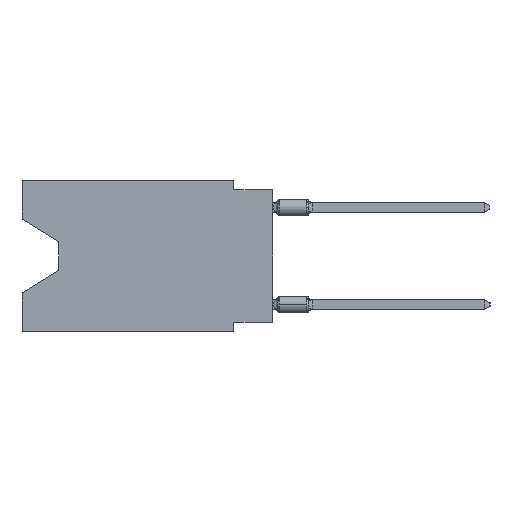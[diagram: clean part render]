
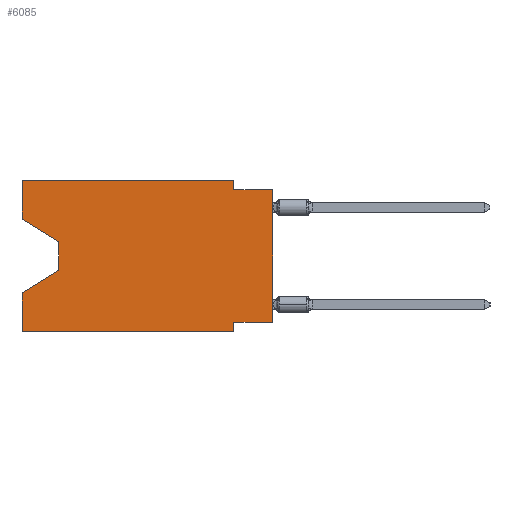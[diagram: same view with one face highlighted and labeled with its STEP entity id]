
A CAD part, left-side view. The second image highlights one B-rep face of the part: STEP entity #6085.
In plain terms, the highlighted planar face has unit normal (-1, 0, 0).
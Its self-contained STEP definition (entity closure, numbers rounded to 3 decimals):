
#552 = AXIS2_PLACEMENT_3D ( 'NONE', #18874, #6855, #30399 ) ;
#792 = EDGE_CURVE ( 'NONE', #24666, #30831, #25590, .T. ) ;
#1021 = CARTESIAN_POINT ( 'NONE',  ( 0., 16.383, -9.906 ) ) ;
#1111 = VERTEX_POINT ( 'NONE', #17667 ) ;
#1192 = VECTOR ( 'NONE', #21020, 1000. ) ;
#1238 = VECTOR ( 'NONE', #3742, 1000. ) ;
#1611 = ORIENTED_EDGE ( 'NONE', *, *, #27553, .F. ) ;
#3358 = DIRECTION ( 'NONE',  ( 0., 0., -1. ) ) ;
#3742 = DIRECTION ( 'NONE',  ( 0., -0.855, -0.519 ) ) ;
#4316 = EDGE_CURVE ( 'NONE', #13164, #8868, #20007, .T. ) ;
#6073 = DIRECTION ( 'NONE',  ( 0., 0., 1. ) ) ;
#6085 = ADVANCED_FACE ( 'NONE', ( #26122 ), #13973, .F. ) ;
#6560 = DIRECTION ( 'NONE',  ( 0., 0.855, -0.519 ) ) ;
#6799 = LINE ( 'NONE', #18811, #1192 ) ;
#6855 = DIRECTION ( 'NONE',  ( 1., 0., 0. ) ) ;
#7568 = VECTOR ( 'NONE', #22548, 1000. ) ;
#8240 = VERTEX_POINT ( 'NONE', #14431 ) ;
#8868 = VERTEX_POINT ( 'NONE', #10588 ) ;
#9000 = VECTOR ( 'NONE', #24006, 1000. ) ;
#9564 = EDGE_CURVE ( 'NONE', #27578, #13164, #17744, .T. ) ;
#9572 = ORIENTED_EDGE ( 'NONE', *, *, #4316, .F. ) ;
#10079 = CARTESIAN_POINT ( 'NONE',  ( 0., 16.383, -7.36 ) ) ;
#10084 = VECTOR ( 'NONE', #27283, 1000. ) ;
#10448 = ORIENTED_EDGE ( 'NONE', *, *, #28836, .T. ) ;
#10464 = DIRECTION ( 'NONE',  ( 0., 1., 0. ) ) ;
#10588 = CARTESIAN_POINT ( 'NONE',  ( 0., 2.54, -9.906 ) ) ;
#11157 = CARTESIAN_POINT ( 'NONE',  ( 0., 2.54, 0. ) ) ;
#11497 = EDGE_LOOP ( 'NONE', ( #19153, #28669, #14744, #1611, #18763, #9572, #24046, #10448, #26878, #20129, #12836, #22927 ) ) ;
#11610 = DIRECTION ( 'NONE',  ( 0., 0., 1. ) ) ;
#11919 = CARTESIAN_POINT ( 'NONE',  ( 0., 2.54, -0.635 ) ) ;
#12631 = CARTESIAN_POINT ( 'NONE',  ( 0., 16.383, 0. ) ) ;
#12836 = ORIENTED_EDGE ( 'NONE', *, *, #30346, .F. ) ;
#13164 = VERTEX_POINT ( 'NONE', #17005 ) ;
#13759 = DIRECTION ( 'NONE',  ( 0., 0., -1. ) ) ;
#13772 = VERTEX_POINT ( 'NONE', #1021 ) ;
#13973 = PLANE ( 'NONE',  #552 ) ;
#14310 = EDGE_CURVE ( 'NONE', #30289, #8240, #6799, .T. ) ;
#14431 = CARTESIAN_POINT ( 'NONE',  ( 0., 16.383, 0. ) ) ;
#14514 = LINE ( 'NONE', #24137, #17975 ) ;
#14744 = ORIENTED_EDGE ( 'NONE', *, *, #18075, .T. ) ;
#15206 = EDGE_CURVE ( 'NONE', #30289, #24666, #27894, .T. ) ;
#15303 = CARTESIAN_POINT ( 'NONE',  ( 0., 16.383, -9.906 ) ) ;
#15611 = LINE ( 'NONE', #15303, #7568 ) ;
#15722 = VECTOR ( 'NONE', #10464, 1000. ) ;
#15878 = CARTESIAN_POINT ( 'NONE',  ( 0., 0., 0. ) ) ;
#16184 = CARTESIAN_POINT ( 'NONE',  ( 0., 0., -9.271 ) ) ;
#16784 = VECTOR ( 'NONE', #13759, 1000. ) ;
#17005 = CARTESIAN_POINT ( 'NONE',  ( 0., 2.54, -9.271 ) ) ;
#17667 = CARTESIAN_POINT ( 'NONE',  ( 0., 0., -0.635 ) ) ;
#17744 = LINE ( 'NONE', #26477, #15722 ) ;
#17975 = VECTOR ( 'NONE', #21774, 1000. ) ;
#18075 = EDGE_CURVE ( 'NONE', #30831, #23262, #25360, .T. ) ;
#18541 = EDGE_CURVE ( 'NONE', #21445, #29987, #24992, .T. ) ;
#18633 = VECTOR ( 'NONE', #3358, 1000. ) ;
#18659 = CARTESIAN_POINT ( 'NONE',  ( 0., 13.97, -5.893 ) ) ;
#18763 = ORIENTED_EDGE ( 'NONE', *, *, #19671, .T. ) ;
#18811 = CARTESIAN_POINT ( 'NONE',  ( 0., 16.383, 0. ) ) ;
#18874 = CARTESIAN_POINT ( 'NONE',  ( 0., 16.383, 0. ) ) ;
#18918 = CARTESIAN_POINT ( 'NONE',  ( 0., 13.97, -4.013 ) ) ;
#19153 = ORIENTED_EDGE ( 'NONE', *, *, #15206, .T. ) ;
#19671 = EDGE_CURVE ( 'NONE', #13772, #8868, #15611, .T. ) ;
#19736 = CARTESIAN_POINT ( 'NONE',  ( 0., 16.383, -2.546 ) ) ;
#20007 = LINE ( 'NONE', #29629, #10084 ) ;
#20129 = ORIENTED_EDGE ( 'NONE', *, *, #18541, .F. ) ;
#20264 = CARTESIAN_POINT ( 'NONE',  ( 0., 2.54, 0. ) ) ;
#20773 = CARTESIAN_POINT ( 'NONE',  ( 0., 13.97, -5.893 ) ) ;
#21020 = DIRECTION ( 'NONE',  ( 0., 0., 1. ) ) ;
#21445 = VERTEX_POINT ( 'NONE', #11157 ) ;
#21774 = DIRECTION ( 'NONE',  ( 0., -1., 0. ) ) ;
#22548 = DIRECTION ( 'NONE',  ( 0., -1., 0. ) ) ;
#22927 = ORIENTED_EDGE ( 'NONE', *, *, #14310, .F. ) ;
#23262 = VERTEX_POINT ( 'NONE', #10079 ) ;
#24006 = DIRECTION ( 'NONE',  ( 0., -1., 0. ) ) ;
#24046 = ORIENTED_EDGE ( 'NONE', *, *, #9564, .F. ) ;
#24137 = CARTESIAN_POINT ( 'NONE',  ( 0., 0., -0.635 ) ) ;
#24666 = VERTEX_POINT ( 'NONE', #18918 ) ;
#24992 = LINE ( 'NONE', #20264, #18633 ) ;
#25349 = LINE ( 'NONE', #28328, #27598 ) ;
#25360 = LINE ( 'NONE', #20773, #28180 ) ;
#25590 = LINE ( 'NONE', #25912, #16784 ) ;
#25693 = CARTESIAN_POINT ( 'NONE',  ( 0., 16.383, -2.546 ) ) ;
#25912 = CARTESIAN_POINT ( 'NONE',  ( 0., 13.97, -4.013 ) ) ;
#26122 = FACE_OUTER_BOUND ( 'NONE', #11497, .T. ) ;
#26477 = CARTESIAN_POINT ( 'NONE',  ( 0., 0., -9.271 ) ) ;
#26878 = ORIENTED_EDGE ( 'NONE', *, *, #28141, .F. ) ;
#27004 = LINE ( 'NONE', #12631, #9000 ) ;
#27082 = VECTOR ( 'NONE', #11610, 1000. ) ;
#27283 = DIRECTION ( 'NONE',  ( 0., 0., -1. ) ) ;
#27553 = EDGE_CURVE ( 'NONE', #13772, #23262, #25349, .T. ) ;
#27578 = VERTEX_POINT ( 'NONE', #16184 ) ;
#27598 = VECTOR ( 'NONE', #6073, 1000. ) ;
#27894 = LINE ( 'NONE', #25693, #1238 ) ;
#28141 = EDGE_CURVE ( 'NONE', #29987, #1111, #14514, .T. ) ;
#28180 = VECTOR ( 'NONE', #6560, 1000. ) ;
#28328 = CARTESIAN_POINT ( 'NONE',  ( 0., 16.383, 0. ) ) ;
#28669 = ORIENTED_EDGE ( 'NONE', *, *, #792, .T. ) ;
#28836 = EDGE_CURVE ( 'NONE', #27578, #1111, #30867, .T. ) ;
#29629 = CARTESIAN_POINT ( 'NONE',  ( 0., 2.54, -9.906 ) ) ;
#29987 = VERTEX_POINT ( 'NONE', #11919 ) ;
#30289 = VERTEX_POINT ( 'NONE', #19736 ) ;
#30346 = EDGE_CURVE ( 'NONE', #8240, #21445, #27004, .T. ) ;
#30399 = DIRECTION ( 'NONE',  ( 0., 0., -1. ) ) ;
#30831 = VERTEX_POINT ( 'NONE', #18659 ) ;
#30867 = LINE ( 'NONE', #15878, #27082 ) ;
